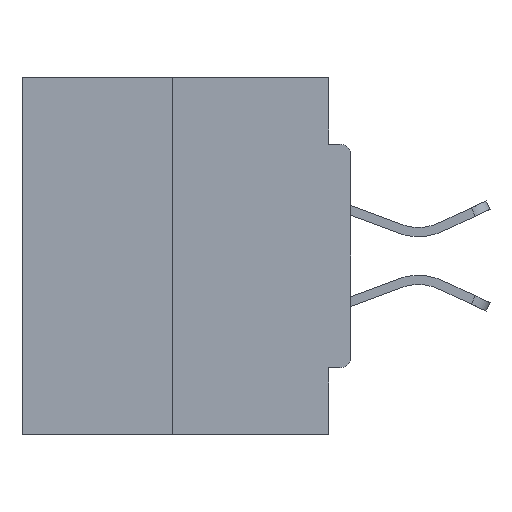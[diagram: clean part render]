
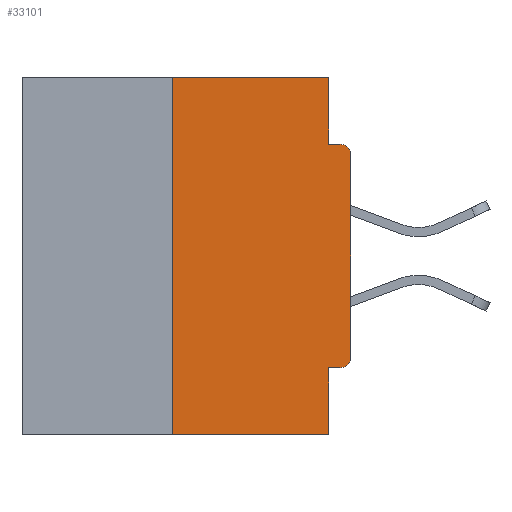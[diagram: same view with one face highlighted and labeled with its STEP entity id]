
A CAD part, left-side view. The second image highlights one B-rep face of the part: STEP entity #33101.
In plain terms, the highlighted planar face has unit normal (-1, 0, 0).
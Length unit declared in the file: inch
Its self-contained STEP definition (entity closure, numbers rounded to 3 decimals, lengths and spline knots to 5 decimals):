
#95 = DIRECTION ( 'NONE',  ( 0., 0., -1. ) ) ;
#263 = CARTESIAN_POINT ( 'NONE',  ( 0., 0.015, -0.1085 ) ) ;
#1051 = DIRECTION ( 'NONE',  ( 0., 0., -1. ) ) ;
#1440 = ORIENTED_EDGE ( 'NONE', *, *, #19593, .F. ) ;
#2120 = ORIENTED_EDGE ( 'NONE', *, *, #7811, .F. ) ;
#2648 = EDGE_CURVE ( 'NONE', #29126, #4498, #32836, .T. ) ;
#3323 = ORIENTED_EDGE ( 'NONE', *, *, #4210, .F. ) ;
#3368 = EDGE_LOOP ( 'NONE', ( #13466, #2120, #4414, #1440, #23397, #26791, #20455, #7093, #3323, #17066 ) ) ;
#3715 = CARTESIAN_POINT ( 'NONE',  ( 0., 0., -0.0935 ) ) ;
#3794 = LINE ( 'NONE', #9402, #15521 ) ;
#4210 = EDGE_CURVE ( 'NONE', #26229, #4498, #25059, .T. ) ;
#4414 = ORIENTED_EDGE ( 'NONE', *, *, #15390, .T. ) ;
#4498 = VERTEX_POINT ( 'NONE', #5080 ) ;
#4787 = VERTEX_POINT ( 'NONE', #20454 ) ;
#5080 = CARTESIAN_POINT ( 'NONE',  ( 0., 0.015, -0.0935 ) ) ;
#6077 = CARTESIAN_POINT ( 'NONE',  ( 0., 0.46, 0. ) ) ;
#6737 = CARTESIAN_POINT ( 'NONE',  ( 0., 0., -0.3915 ) ) ;
#7093 = ORIENTED_EDGE ( 'NONE', *, *, #2648, .T. ) ;
#7317 = LINE ( 'NONE', #17984, #29430 ) ;
#7811 = EDGE_CURVE ( 'NONE', #15235, #9254, #7317, .T. ) ;
#8176 = AXIS2_PLACEMENT_3D ( 'NONE', #17542, #15452, #33859 ) ;
#9254 = VERTEX_POINT ( 'NONE', #12343 ) ;
#9386 = VECTOR ( 'NONE', #16376, 39.37008 ) ;
#9402 = CARTESIAN_POINT ( 'NONE',  ( 0., 0.031, 0. ) ) ;
#9429 = LINE ( 'NONE', #24984, #10262 ) ;
#9727 = VECTOR ( 'NONE', #22507, 39.37008 ) ;
#10262 = VECTOR ( 'NONE', #1051, 39.37008 ) ;
#10644 = LINE ( 'NONE', #21276, #9386 ) ;
#10800 = VERTEX_POINT ( 'NONE', #12804 ) ;
#11058 = AXIS2_PLACEMENT_3D ( 'NONE', #6077, #17082, #25481 ) ;
#12343 = CARTESIAN_POINT ( 'NONE',  ( 0., 0.25, 0. ) ) ;
#12746 = DIRECTION ( 'NONE',  ( 0., -1., 0. ) ) ;
#12804 = CARTESIAN_POINT ( 'NONE',  ( 0., 0.031, -0.4065 ) ) ;
#13217 = VECTOR ( 'NONE', #26971, 39.37008 ) ;
#13466 = ORIENTED_EDGE ( 'NONE', *, *, #33038, .F. ) ;
#15206 = DIRECTION ( 'NONE',  ( 0., 0., 1. ) ) ;
#15235 = VERTEX_POINT ( 'NONE', #22515 ) ;
#15309 = VECTOR ( 'NONE', #20962, 39.37008 ) ;
#15390 = EDGE_CURVE ( 'NONE', #15235, #24379, #25853, .T. ) ;
#15452 = DIRECTION ( 'NONE',  ( -1., 0., 0. ) ) ;
#15521 = VECTOR ( 'NONE', #22335, 39.37008 ) ;
#16376 = DIRECTION ( 'NONE',  ( 0., -1., 0. ) ) ;
#17066 = ORIENTED_EDGE ( 'NONE', *, *, #33078, .F. ) ;
#17082 = DIRECTION ( 'NONE',  ( 1., 0., 0. ) ) ;
#17107 = CARTESIAN_POINT ( 'NONE',  ( 0., 0., -0.4065 ) ) ;
#17542 = CARTESIAN_POINT ( 'NONE',  ( 0., 0.015, -0.3915 ) ) ;
#17692 = VERTEX_POINT ( 'NONE', #29333 ) ;
#17722 = AXIS2_PLACEMENT_3D ( 'NONE', #263, #24395, #95 ) ;
#17984 = CARTESIAN_POINT ( 'NONE',  ( 0., 0.25, 0. ) ) ;
#19593 = EDGE_CURVE ( 'NONE', #10800, #24379, #9429, .T. ) ;
#19608 = EDGE_CURVE ( 'NONE', #17692, #10800, #28114, .T. ) ;
#20454 = CARTESIAN_POINT ( 'NONE',  ( 0., 0.031, 0. ) ) ;
#20455 = ORIENTED_EDGE ( 'NONE', *, *, #27882, .T. ) ;
#20962 = DIRECTION ( 'NONE',  ( 0., 0., 1. ) ) ;
#21276 = CARTESIAN_POINT ( 'NONE',  ( 0., 0.46, 0. ) ) ;
#22335 = DIRECTION ( 'NONE',  ( 0., 0., -1. ) ) ;
#22507 = DIRECTION ( 'NONE',  ( 0., 1., 0. ) ) ;
#22515 = CARTESIAN_POINT ( 'NONE',  ( 0., 0.25, -0.5 ) ) ;
#23397 = ORIENTED_EDGE ( 'NONE', *, *, #19608, .F. ) ;
#24379 = VERTEX_POINT ( 'NONE', #28670 ) ;
#24395 = DIRECTION ( 'NONE',  ( -1., 0., 0. ) ) ;
#24984 = CARTESIAN_POINT ( 'NONE',  ( 0., 0.031, -0.5 ) ) ;
#25059 = LINE ( 'NONE', #3715, #13217 ) ;
#25481 = DIRECTION ( 'NONE',  ( 0., 0., -1. ) ) ;
#25853 = LINE ( 'NONE', #31448, #31296 ) ;
#26229 = VERTEX_POINT ( 'NONE', #27649 ) ;
#26791 = ORIENTED_EDGE ( 'NONE', *, *, #32446, .T. ) ;
#26971 = DIRECTION ( 'NONE',  ( 0., -1., 0. ) ) ;
#27649 = CARTESIAN_POINT ( 'NONE',  ( 0., 0.031, -0.0935 ) ) ;
#27775 = FACE_OUTER_BOUND ( 'NONE', #3368, .T. ) ;
#27882 = EDGE_CURVE ( 'NONE', #28656, #29126, #34492, .T. ) ;
#28092 = PLANE ( 'NONE',  #11058 ) ;
#28114 = LINE ( 'NONE', #17107, #9727 ) ;
#28656 = VERTEX_POINT ( 'NONE', #6737 ) ;
#28670 = CARTESIAN_POINT ( 'NONE',  ( 0., 0.031, -0.5 ) ) ;
#29126 = VERTEX_POINT ( 'NONE', #31529 ) ;
#29333 = CARTESIAN_POINT ( 'NONE',  ( 0., 0.015, -0.4065 ) ) ;
#29430 = VECTOR ( 'NONE', #15206, 39.37008 ) ;
#31296 = VECTOR ( 'NONE', #12746, 39.37008 ) ;
#31448 = CARTESIAN_POINT ( 'NONE',  ( 0., 0.46, -0.5 ) ) ;
#31529 = CARTESIAN_POINT ( 'NONE',  ( 0., 0., -0.1085 ) ) ;
#32232 = CIRCLE ( 'NONE', #8176, 0.015 ) ;
#32446 = EDGE_CURVE ( 'NONE', #17692, #28656, #32232, .T. ) ;
#32836 = CIRCLE ( 'NONE', #17722, 0.015 ) ;
#33038 = EDGE_CURVE ( 'NONE', #9254, #4787, #10644, .T. ) ;
#33078 = EDGE_CURVE ( 'NONE', #4787, #26229, #3794, .T. ) ;
#33101 = ADVANCED_FACE ( 'NONE', ( #27775 ), #28092, .F. ) ;
#33859 = DIRECTION ( 'NONE',  ( 0., 0., -1. ) ) ;
#34308 = CARTESIAN_POINT ( 'NONE',  ( 0., 0., 0. ) ) ;
#34492 = LINE ( 'NONE', #34308, #15309 ) ;
